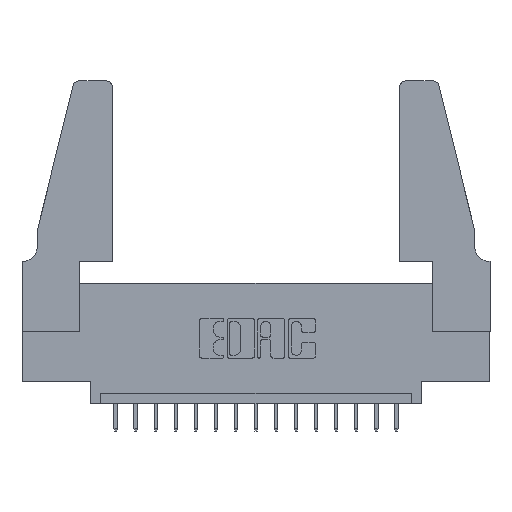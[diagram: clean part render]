
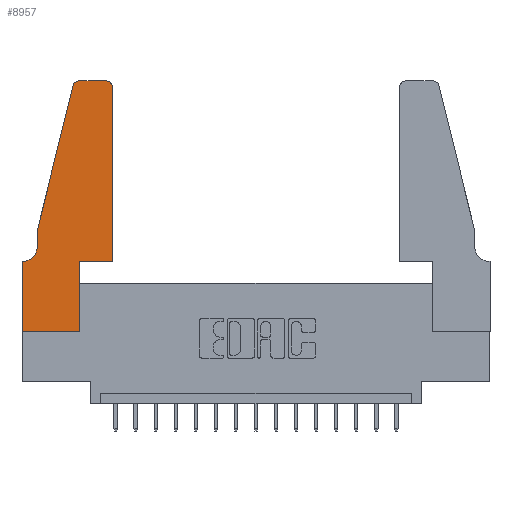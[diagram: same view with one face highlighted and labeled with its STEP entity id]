
A CAD part, top view. The second image highlights one B-rep face of the part: STEP entity #8957.
In plain terms, the highlighted planar face has unit normal (0, 0, 1).
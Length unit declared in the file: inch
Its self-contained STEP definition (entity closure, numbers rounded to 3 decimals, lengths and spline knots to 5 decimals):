
#761 = EDGE_CURVE ( 'NONE', #16005, #12020, #3008, .T. ) ;
#981 = CARTESIAN_POINT ( 'NONE',  ( 0., 0., 0.37 ) ) ;
#1121 = DIRECTION ( 'NONE',  ( 0., 1., 0. ) ) ;
#1283 = VERTEX_POINT ( 'NONE', #10421 ) ;
#1399 = VERTEX_POINT ( 'NONE', #3003 ) ;
#1581 = CARTESIAN_POINT ( 'NONE',  ( 0., 0.35, 0.37 ) ) ;
#1654 = DIRECTION ( 'NONE',  ( 1., 0., 0. ) ) ;
#1718 = CARTESIAN_POINT ( 'NONE',  ( 0.2865, 0., 0.37 ) ) ;
#2004 = LINE ( 'NONE', #3250, #13961 ) ;
#2134 = CARTESIAN_POINT ( 'NONE',  ( 0.4205, 1.22, 0.37 ) ) ;
#2179 = DIRECTION ( 'NONE',  ( 1., 0., 0. ) ) ;
#2344 = VECTOR ( 'NONE', #17256, 39.37008 ) ;
#2353 = CARTESIAN_POINT ( 'NONE',  ( 0.284, 1.22, 0.37 ) ) ;
#2389 = DIRECTION ( 'NONE',  ( 0., 0., 1. ) ) ;
#2394 = VECTOR ( 'NONE', #1121, 39.37008 ) ;
#2499 = CARTESIAN_POINT ( 'NONE',  ( 0.4505, 1.22, 0.37 ) ) ;
#2595 = VECTOR ( 'NONE', #14529, 39.37008 ) ;
#2669 = EDGE_CURVE ( 'NONE', #9426, #3050, #8167, .T. ) ;
#2985 = EDGE_CURVE ( 'NONE', #1399, #3826, #6702, .T. ) ;
#3003 = CARTESIAN_POINT ( 'NONE',  ( 0.0755, 0.42, 0.37 ) ) ;
#3008 = CIRCLE ( 'NONE', #4124, 0.03 ) ;
#3050 = VERTEX_POINT ( 'NONE', #16298 ) ;
#3083 = CARTESIAN_POINT ( 'NONE',  ( 0., 0., 0.37 ) ) ;
#3250 = CARTESIAN_POINT ( 'NONE',  ( 0.0755, 0.5, 0.37 ) ) ;
#3318 = EDGE_CURVE ( 'NONE', #17191, #16005, #15670, .T. ) ;
#3445 = CIRCLE ( 'NONE', #12646, 0.03 ) ;
#3513 = DIRECTION ( 'NONE',  ( 0., 0., 1. ) ) ;
#3826 = VERTEX_POINT ( 'NONE', #7991 ) ;
#3991 = EDGE_LOOP ( 'NONE', ( #4892, #14382, #13494, #5283, #7457, #12804, #10127, #9312, #6565, #4528, #4324, #13787 ) ) ;
#4124 = AXIS2_PLACEMENT_3D ( 'NONE', #2353, #7641, #15903 ) ;
#4324 = ORIENTED_EDGE ( 'NONE', *, *, #13602, .T. ) ;
#4528 = ORIENTED_EDGE ( 'NONE', *, *, #11196, .T. ) ;
#4832 = PLANE ( 'NONE',  #13698 ) ;
#4892 = ORIENTED_EDGE ( 'NONE', *, *, #3318, .T. ) ;
#5122 = CARTESIAN_POINT ( 'NONE',  ( 0.4505, 0.35, 0.37 ) ) ;
#5225 = VERTEX_POINT ( 'NONE', #16363 ) ;
#5283 = ORIENTED_EDGE ( 'NONE', *, *, #16251, .T. ) ;
#5479 = DIRECTION ( 'NONE',  ( -1., 0., 0. ) ) ;
#5487 = VERTEX_POINT ( 'NONE', #10717 ) ;
#5866 = AXIS2_PLACEMENT_3D ( 'NONE', #6705, #12276, #5479 ) ;
#6231 = DIRECTION ( 'NONE',  ( -0.239, -0.971, 0. ) ) ;
#6262 = LINE ( 'NONE', #981, #10745 ) ;
#6565 = ORIENTED_EDGE ( 'NONE', *, *, #2669, .T. ) ;
#6702 = CIRCLE ( 'NONE', #5866, 0.07 ) ;
#6705 = CARTESIAN_POINT ( 'NONE',  ( 0.0055, 0.42, 0.37 ) ) ;
#6924 = EDGE_CURVE ( 'NONE', #12020, #5225, #2004, .T. ) ;
#7457 = ORIENTED_EDGE ( 'NONE', *, *, #2985, .T. ) ;
#7641 = DIRECTION ( 'NONE',  ( 0., 0., 1. ) ) ;
#7655 = DIRECTION ( 'NONE',  ( -1., 0., 0. ) ) ;
#7991 = CARTESIAN_POINT ( 'NONE',  ( 0.0055, 0.35, 0.37 ) ) ;
#8167 = LINE ( 'NONE', #13391, #2394 ) ;
#8570 = DIRECTION ( 'NONE',  ( 0., -1., 0. ) ) ;
#8957 = ADVANCED_FACE ( 'NONE', ( #16804 ), #4832, .T. ) ;
#8958 = LINE ( 'NONE', #16898, #13232 ) ;
#9065 = DIRECTION ( 'NONE',  ( 1., 0., 0. ) ) ;
#9312 = ORIENTED_EDGE ( 'NONE', *, *, #14546, .T. ) ;
#9426 = VERTEX_POINT ( 'NONE', #1718 ) ;
#9660 = LINE ( 'NONE', #3083, #14560 ) ;
#9879 = CARTESIAN_POINT ( 'NONE',  ( 0.0755, 0.5, 0.37 ) ) ;
#9967 = LINE ( 'NONE', #9879, #11303 ) ;
#10127 = ORIENTED_EDGE ( 'NONE', *, *, #11238, .T. ) ;
#10421 = CARTESIAN_POINT ( 'NONE',  ( 0.4505, 0.35, 0.37 ) ) ;
#10562 = CARTESIAN_POINT ( 'NONE',  ( 0.4205, 1.25, 0.37 ) ) ;
#10717 = CARTESIAN_POINT ( 'NONE',  ( 0., 0., 0.37 ) ) ;
#10745 = VECTOR ( 'NONE', #9065, 39.37008 ) ;
#11196 = EDGE_CURVE ( 'NONE', #3050, #1283, #16278, .T. ) ;
#11238 = EDGE_CURVE ( 'NONE', #14691, #5487, #9660, .T. ) ;
#11303 = VECTOR ( 'NONE', #8570, 39.37008 ) ;
#12020 = VERTEX_POINT ( 'NONE', #12894 ) ;
#12023 = EDGE_CURVE ( 'NONE', #15577, #17191, #3445, .T. ) ;
#12276 = DIRECTION ( 'NONE',  ( 0., 0., -1. ) ) ;
#12646 = AXIS2_PLACEMENT_3D ( 'NONE', #2134, #2389, #13069 ) ;
#12804 = ORIENTED_EDGE ( 'NONE', *, *, #13022, .T. ) ;
#12894 = CARTESIAN_POINT ( 'NONE',  ( 0.25487, 1.22718, 0.37 ) ) ;
#13022 = EDGE_CURVE ( 'NONE', #3826, #14691, #8958, .T. ) ;
#13069 = DIRECTION ( 'NONE',  ( 1., 0., 0. ) ) ;
#13232 = VECTOR ( 'NONE', #7655, 39.37008 ) ;
#13391 = CARTESIAN_POINT ( 'NONE',  ( 0.2865, 0.35, 0.37 ) ) ;
#13494 = ORIENTED_EDGE ( 'NONE', *, *, #6924, .T. ) ;
#13602 = EDGE_CURVE ( 'NONE', #1283, #15577, #15848, .T. ) ;
#13698 = AXIS2_PLACEMENT_3D ( 'NONE', #15461, #3513, #2179 ) ;
#13787 = ORIENTED_EDGE ( 'NONE', *, *, #12023, .T. ) ;
#13961 = VECTOR ( 'NONE', #6231, 39.37008 ) ;
#14009 = CARTESIAN_POINT ( 'NONE',  ( 0.4505, 0.35, 0.37 ) ) ;
#14382 = ORIENTED_EDGE ( 'NONE', *, *, #761, .T. ) ;
#14529 = DIRECTION ( 'NONE',  ( -1., 0., 0. ) ) ;
#14546 = EDGE_CURVE ( 'NONE', #5487, #9426, #6262, .T. ) ;
#14560 = VECTOR ( 'NONE', #14958, 39.37008 ) ;
#14691 = VERTEX_POINT ( 'NONE', #1581 ) ;
#14958 = DIRECTION ( 'NONE',  ( 0., -1., 0. ) ) ;
#15401 = VECTOR ( 'NONE', #1654, 39.37008 ) ;
#15461 = CARTESIAN_POINT ( 'NONE',  ( 0., 0.35, 0.37 ) ) ;
#15570 = CARTESIAN_POINT ( 'NONE',  ( 0.284, 1.25, 0.37 ) ) ;
#15577 = VERTEX_POINT ( 'NONE', #2499 ) ;
#15670 = LINE ( 'NONE', #17088, #2595 ) ;
#15848 = LINE ( 'NONE', #5122, #2344 ) ;
#15903 = DIRECTION ( 'NONE',  ( 1., 0., 0. ) ) ;
#16005 = VERTEX_POINT ( 'NONE', #15570 ) ;
#16251 = EDGE_CURVE ( 'NONE', #5225, #1399, #9967, .T. ) ;
#16278 = LINE ( 'NONE', #14009, #15401 ) ;
#16298 = CARTESIAN_POINT ( 'NONE',  ( 0.2865, 0.35, 0.37 ) ) ;
#16363 = CARTESIAN_POINT ( 'NONE',  ( 0.0755, 0.5, 0.37 ) ) ;
#16804 = FACE_OUTER_BOUND ( 'NONE', #3991, .T. ) ;
#16898 = CARTESIAN_POINT ( 'NONE',  ( 0.0755, 0.35, 0.37 ) ) ;
#17088 = CARTESIAN_POINT ( 'NONE',  ( 0.2605, 1.25, 0.37 ) ) ;
#17191 = VERTEX_POINT ( 'NONE', #10562 ) ;
#17256 = DIRECTION ( 'NONE',  ( 0., 1., 0. ) ) ;
